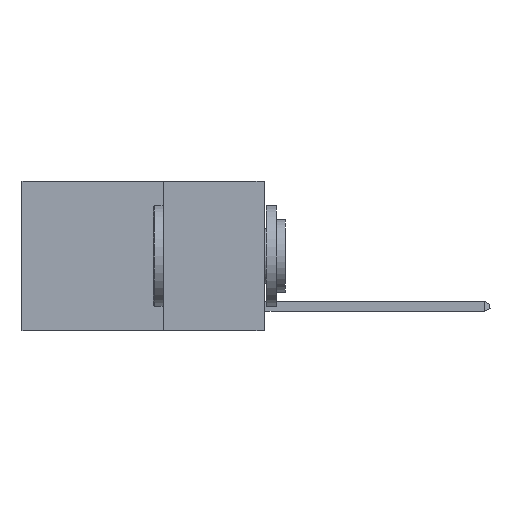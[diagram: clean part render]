
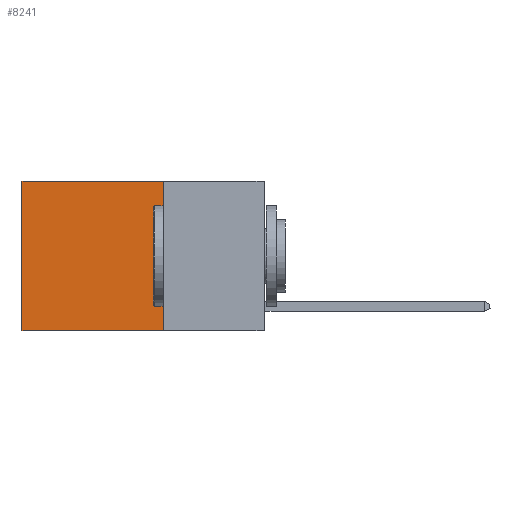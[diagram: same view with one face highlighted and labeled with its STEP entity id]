
A CAD part, left-side view. The second image highlights one B-rep face of the part: STEP entity #8241.
In plain terms, the highlighted planar face has unit normal (-1, 0, 0).
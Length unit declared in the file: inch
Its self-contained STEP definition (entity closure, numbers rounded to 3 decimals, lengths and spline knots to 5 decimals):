
#88 = FACE_OUTER_BOUND ( 'NONE', #5674, .T. ) ;
#124 = EDGE_CURVE ( 'NONE', #24788, #16990, #17320, .T. ) ;
#2760 = CARTESIAN_POINT ( 'NONE',  ( 0.2625, 0.25, 0. ) ) ;
#2916 = CARTESIAN_POINT ( 'NONE',  ( 0.2625, 0.6, 0. ) ) ;
#3951 = ORIENTED_EDGE ( 'NONE', *, *, #18135, .T. ) ;
#4338 = LINE ( 'NONE', #13876, #11456 ) ;
#5674 = EDGE_LOOP ( 'NONE', ( #3951, #16908, #13459, #16783 ) ) ;
#6492 = LINE ( 'NONE', #24067, #15131 ) ;
#6615 = DIRECTION ( 'NONE',  ( 0., 0., -1. ) ) ;
#6834 = CARTESIAN_POINT ( 'NONE',  ( 0.2625, 0.25, 0. ) ) ;
#7524 = DIRECTION ( 'NONE',  ( 0., 1., 0. ) ) ;
#8241 = ADVANCED_FACE ( 'NONE', ( #88 ), #11604, .F. ) ;
#8347 = VECTOR ( 'NONE', #16414, 39.37008 ) ;
#8651 = LINE ( 'NONE', #2916, #8347 ) ;
#9525 = EDGE_CURVE ( 'NONE', #18108, #15919, #4338, .T. ) ;
#10059 = EDGE_CURVE ( 'NONE', #24788, #18108, #6492, .T. ) ;
#11456 = VECTOR ( 'NONE', #12224, 39.37008 ) ;
#11604 = PLANE ( 'NONE',  #13831 ) ;
#11850 = DIRECTION ( 'NONE',  ( 0., 0., -1. ) ) ;
#12224 = DIRECTION ( 'NONE',  ( 0., 1., 0. ) ) ;
#13143 = CARTESIAN_POINT ( 'NONE',  ( 0.2625, 0.6, -0.37 ) ) ;
#13459 = ORIENTED_EDGE ( 'NONE', *, *, #10059, .F. ) ;
#13589 = CARTESIAN_POINT ( 'NONE',  ( 0.2625, 0.25, 0. ) ) ;
#13831 = AXIS2_PLACEMENT_3D ( 'NONE', #2760, #23339, #11850 ) ;
#13876 = CARTESIAN_POINT ( 'NONE',  ( 0.2625, 0.25, -0.37 ) ) ;
#14928 = VECTOR ( 'NONE', #7524, 39.37008 ) ;
#15131 = VECTOR ( 'NONE', #6615, 39.37008 ) ;
#15919 = VERTEX_POINT ( 'NONE', #13143 ) ;
#16414 = DIRECTION ( 'NONE',  ( 0., 0., -1. ) ) ;
#16783 = ORIENTED_EDGE ( 'NONE', *, *, #124, .T. ) ;
#16908 = ORIENTED_EDGE ( 'NONE', *, *, #9525, .F. ) ;
#16990 = VERTEX_POINT ( 'NONE', #25187 ) ;
#17320 = LINE ( 'NONE', #13589, #14928 ) ;
#18108 = VERTEX_POINT ( 'NONE', #22810 ) ;
#18135 = EDGE_CURVE ( 'NONE', #16990, #15919, #8651, .T. ) ;
#22810 = CARTESIAN_POINT ( 'NONE',  ( 0.2625, 0.25, -0.37 ) ) ;
#23339 = DIRECTION ( 'NONE',  ( 1., 0., 0. ) ) ;
#24067 = CARTESIAN_POINT ( 'NONE',  ( 0.2625, 0.25, 0. ) ) ;
#24788 = VERTEX_POINT ( 'NONE', #6834 ) ;
#25187 = CARTESIAN_POINT ( 'NONE',  ( 0.2625, 0.6, 0. ) ) ;
